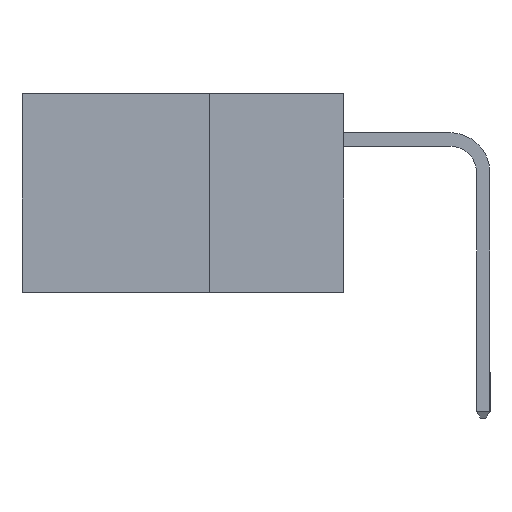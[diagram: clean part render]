
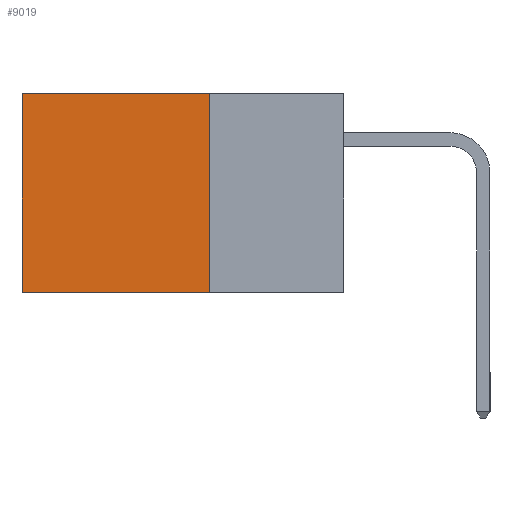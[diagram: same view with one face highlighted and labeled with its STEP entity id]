
A CAD part, left-side view. The second image highlights one B-rep face of the part: STEP entity #9019.
In plain terms, the highlighted planar face has unit normal (-1, 0, 0).
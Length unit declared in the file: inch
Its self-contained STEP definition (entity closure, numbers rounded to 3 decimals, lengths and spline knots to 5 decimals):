
#76 = CARTESIAN_POINT ( 'NONE',  ( 0.298, 0.25, -0.37 ) ) ;
#607 = LINE ( 'NONE', #11271, #3251 ) ;
#776 = DIRECTION ( 'NONE',  ( 0., 1., 0. ) ) ;
#942 = VERTEX_POINT ( 'NONE', #9111 ) ;
#1001 = LINE ( 'NONE', #13245, #3692 ) ;
#1121 = CARTESIAN_POINT ( 'NONE',  ( 0.298, 0.6, 0. ) ) ;
#1386 = ORIENTED_EDGE ( 'NONE', *, *, #5250, .F. ) ;
#1551 = VERTEX_POINT ( 'NONE', #76 ) ;
#2069 = ORIENTED_EDGE ( 'NONE', *, *, #11467, .T. ) ;
#2310 = CARTESIAN_POINT ( 'NONE',  ( 0.298, 0.25, 0. ) ) ;
#2389 = DIRECTION ( 'NONE',  ( 0., 0., -1. ) ) ;
#2725 = VERTEX_POINT ( 'NONE', #4594 ) ;
#2971 = AXIS2_PLACEMENT_3D ( 'NONE', #7994, #4696, #9216 ) ;
#3251 = VECTOR ( 'NONE', #9026, 39.37008 ) ;
#3459 = ORIENTED_EDGE ( 'NONE', *, *, #6585, .T. ) ;
#3692 = VECTOR ( 'NONE', #776, 39.37008 ) ;
#3736 = ORIENTED_EDGE ( 'NONE', *, *, #4019, .F. ) ;
#4019 = EDGE_CURVE ( 'NONE', #12617, #1551, #8271, .T. ) ;
#4594 = CARTESIAN_POINT ( 'NONE',  ( 0.298, 0.6, 0. ) ) ;
#4696 = DIRECTION ( 'NONE',  ( 1., 0., 0. ) ) ;
#5250 = EDGE_CURVE ( 'NONE', #1551, #942, #607, .T. ) ;
#5949 = VECTOR ( 'NONE', #14369, 39.37008 ) ;
#6585 = EDGE_CURVE ( 'NONE', #12617, #2725, #1001, .T. ) ;
#7326 = FACE_OUTER_BOUND ( 'NONE', #8712, .T. ) ;
#7994 = CARTESIAN_POINT ( 'NONE',  ( 0.298, 0.25, 0. ) ) ;
#8271 = LINE ( 'NONE', #13316, #5949 ) ;
#8622 = LINE ( 'NONE', #1121, #8965 ) ;
#8712 = EDGE_LOOP ( 'NONE', ( #2069, #1386, #3736, #3459 ) ) ;
#8965 = VECTOR ( 'NONE', #2389, 39.37008 ) ;
#9019 = ADVANCED_FACE ( 'NONE', ( #7326 ), #12423, .F. ) ;
#9026 = DIRECTION ( 'NONE',  ( 0., 1., 0. ) ) ;
#9111 = CARTESIAN_POINT ( 'NONE',  ( 0.298, 0.6, -0.37 ) ) ;
#9216 = DIRECTION ( 'NONE',  ( 0., 0., -1. ) ) ;
#11271 = CARTESIAN_POINT ( 'NONE',  ( 0.298, 0.25, -0.37 ) ) ;
#11467 = EDGE_CURVE ( 'NONE', #2725, #942, #8622, .T. ) ;
#12423 = PLANE ( 'NONE',  #2971 ) ;
#12617 = VERTEX_POINT ( 'NONE', #2310 ) ;
#13245 = CARTESIAN_POINT ( 'NONE',  ( 0.298, 0.25, 0. ) ) ;
#13316 = CARTESIAN_POINT ( 'NONE',  ( 0.298, 0.25, 0. ) ) ;
#14369 = DIRECTION ( 'NONE',  ( 0., 0., -1. ) ) ;
